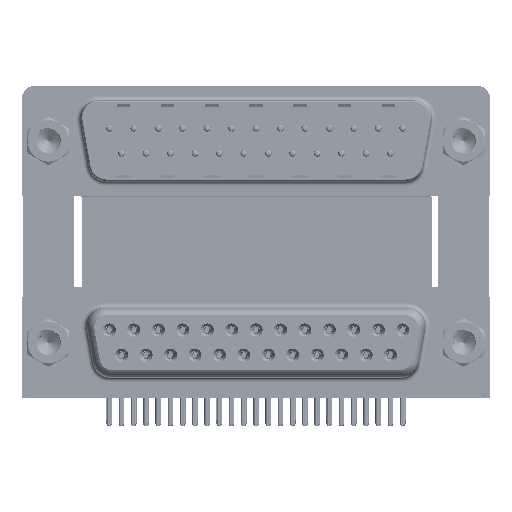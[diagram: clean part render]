
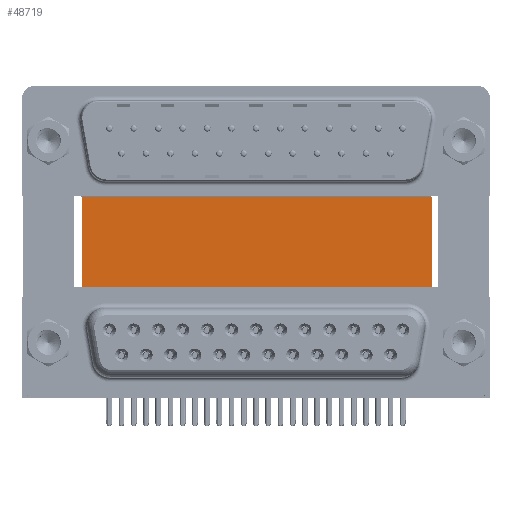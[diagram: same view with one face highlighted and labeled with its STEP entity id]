
A CAD part, top view. The second image highlights one B-rep face of the part: STEP entity #48719.
In plain terms, the highlighted planar face has unit normal (0, 0, 1).
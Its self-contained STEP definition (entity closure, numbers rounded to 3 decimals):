
#333 = ORIENTED_EDGE ( 'NONE', *, *, #56336, .F. ) ;
#1044 = LINE ( 'NONE', #42969, #1749 ) ;
#1749 = VECTOR ( 'NONE', #20625, 1000. ) ;
#2341 = EDGE_LOOP ( 'NONE', ( #59388, #333, #40086, #31749 ) ) ;
#3531 = CARTESIAN_POINT ( 'NONE',  ( 3.79, -3.735, -12. ) ) ;
#5370 = VERTEX_POINT ( 'NONE', #55927 ) ;
#6403 = VERTEX_POINT ( 'NONE', #56224 ) ;
#6644 = CARTESIAN_POINT ( 'NONE',  ( 43.43, 16.585, -12. ) ) ;
#10836 = DIRECTION ( 'NONE',  ( -1., 0., 0. ) ) ;
#14726 = VECTOR ( 'NONE', #58555, 1000. ) ;
#15261 = CARTESIAN_POINT ( 'NONE',  ( 3.79, 16.585, -12. ) ) ;
#17912 = VERTEX_POINT ( 'NONE', #3531 ) ;
#20527 = EDGE_CURVE ( 'NONE', #53839, #17912, #56665, .T. ) ;
#20625 = DIRECTION ( 'NONE',  ( 1., 0., 0. ) ) ;
#23307 = EDGE_CURVE ( 'NONE', #53839, #5370, #59149, .T. ) ;
#24724 = PLANE ( 'NONE',  #40374 ) ;
#28981 = CARTESIAN_POINT ( 'NONE',  ( 3.79, 16.585, -12. ) ) ;
#29555 = FACE_OUTER_BOUND ( 'NONE', #2341, .T. ) ;
#31749 = ORIENTED_EDGE ( 'NONE', *, *, #20527, .T. ) ;
#32232 = CARTESIAN_POINT ( 'NONE',  ( 3.79, 16.585, -12. ) ) ;
#34143 = DIRECTION ( 'NONE',  ( 0., -1., 0. ) ) ;
#35368 = EDGE_CURVE ( 'NONE', #17912, #6403, #1044, .T. ) ;
#37050 = DIRECTION ( 'NONE',  ( 0., -1., 0. ) ) ;
#40086 = ORIENTED_EDGE ( 'NONE', *, *, #23307, .F. ) ;
#40374 = AXIS2_PLACEMENT_3D ( 'NONE', #28981, #43150, #10836 ) ;
#41009 = CARTESIAN_POINT ( 'NONE',  ( 3.79, 16.585, -12. ) ) ;
#42969 = CARTESIAN_POINT ( 'NONE',  ( 3.79, -3.735, -12. ) ) ;
#43150 = DIRECTION ( 'NONE',  ( 0., 0., -1. ) ) ;
#43800 = LINE ( 'NONE', #6644, #43832 ) ;
#43832 = VECTOR ( 'NONE', #34143, 1000. ) ;
#48719 = ADVANCED_FACE ( 'NONE', ( #29555 ), #24724, .F. ) ;
#53246 = VECTOR ( 'NONE', #37050, 1000. ) ;
#53839 = VERTEX_POINT ( 'NONE', #32232 ) ;
#55927 = CARTESIAN_POINT ( 'NONE',  ( 43.43, 16.585, -12. ) ) ;
#56224 = CARTESIAN_POINT ( 'NONE',  ( 43.43, -3.735, -12. ) ) ;
#56336 = EDGE_CURVE ( 'NONE', #5370, #6403, #43800, .T. ) ;
#56665 = LINE ( 'NONE', #15261, #53246 ) ;
#58555 = DIRECTION ( 'NONE',  ( 1., 0., 0. ) ) ;
#59149 = LINE ( 'NONE', #41009, #14726 ) ;
#59388 = ORIENTED_EDGE ( 'NONE', *, *, #35368, .T. ) ;
